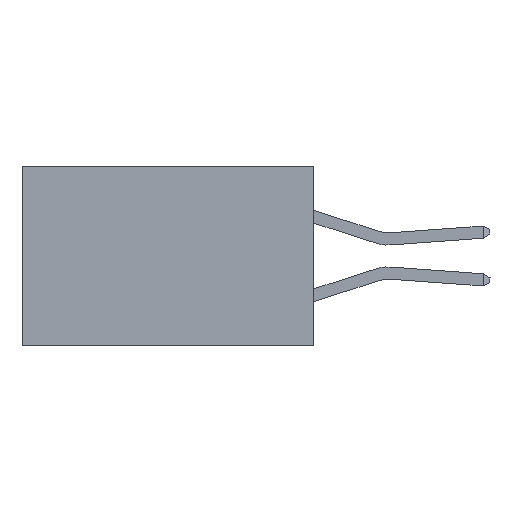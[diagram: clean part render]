
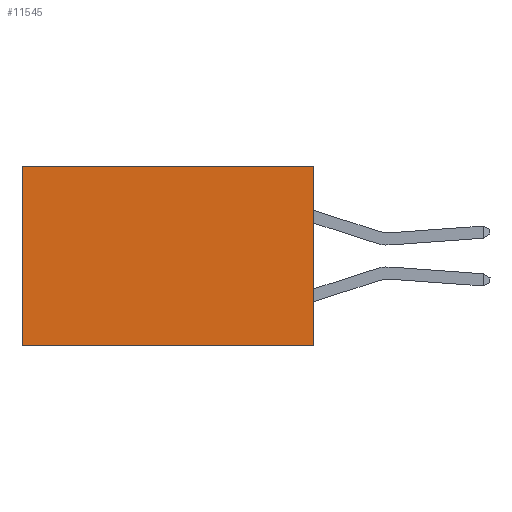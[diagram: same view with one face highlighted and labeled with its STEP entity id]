
A CAD part, left-side view. The second image highlights one B-rep face of the part: STEP entity #11545.
In plain terms, the highlighted planar face has unit normal (-1, 0, 0).
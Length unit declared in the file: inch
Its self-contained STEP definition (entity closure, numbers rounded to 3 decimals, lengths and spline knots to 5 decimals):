
#712 = ORIENTED_EDGE ( 'NONE', *, *, #10386, .T. ) ;
#1958 = CARTESIAN_POINT ( 'NONE',  ( 0.2875, 0.6, 0. ) ) ;
#3313 = ORIENTED_EDGE ( 'NONE', *, *, #13810, .F. ) ;
#3644 = LINE ( 'NONE', #19814, #23081 ) ;
#4538 = VECTOR ( 'NONE', #5929, 39.37008 ) ;
#5320 = DIRECTION ( 'NONE',  ( 1., 0., 0. ) ) ;
#5450 = ORIENTED_EDGE ( 'NONE', *, *, #22637, .T. ) ;
#5929 = DIRECTION ( 'NONE',  ( 0., 0., -1. ) ) ;
#6014 = CARTESIAN_POINT ( 'NONE',  ( 0.2875, 0., 0. ) ) ;
#7818 = EDGE_CURVE ( 'NONE', #17699, #22112, #12250, .T. ) ;
#9010 = DIRECTION ( 'NONE',  ( 0., 1., 0. ) ) ;
#10386 = EDGE_CURVE ( 'NONE', #18219, #22112, #10652, .T. ) ;
#10652 = LINE ( 'NONE', #1958, #19691 ) ;
#11545 = ADVANCED_FACE ( 'NONE', ( #23475 ), #21593, .F. ) ;
#11817 = DIRECTION ( 'NONE',  ( 0., 1., 0. ) ) ;
#12250 = LINE ( 'NONE', #22729, #16512 ) ;
#12575 = VERTEX_POINT ( 'NONE', #23031 ) ;
#12953 = CARTESIAN_POINT ( 'NONE',  ( 0.2875, 0., -0.37 ) ) ;
#13810 = EDGE_CURVE ( 'NONE', #12575, #17699, #17866, .T. ) ;
#14348 = CARTESIAN_POINT ( 'NONE',  ( 0.2875, 0., 0. ) ) ;
#15275 = ORIENTED_EDGE ( 'NONE', *, *, #7818, .F. ) ;
#16512 = VECTOR ( 'NONE', #11817, 39.37008 ) ;
#16544 = DIRECTION ( 'NONE',  ( 0., 0., -1. ) ) ;
#17699 = VERTEX_POINT ( 'NONE', #12953 ) ;
#17785 = AXIS2_PLACEMENT_3D ( 'NONE', #14348, #5320, #17991 ) ;
#17866 = LINE ( 'NONE', #6014, #4538 ) ;
#17991 = DIRECTION ( 'NONE',  ( 0., 0., -1. ) ) ;
#18219 = VERTEX_POINT ( 'NONE', #23655 ) ;
#19522 = CARTESIAN_POINT ( 'NONE',  ( 0.2875, 0.6, -0.37 ) ) ;
#19691 = VECTOR ( 'NONE', #16544, 39.37008 ) ;
#19718 = EDGE_LOOP ( 'NONE', ( #712, #15275, #3313, #5450 ) ) ;
#19814 = CARTESIAN_POINT ( 'NONE',  ( 0.2875, 0., 0. ) ) ;
#21593 = PLANE ( 'NONE',  #17785 ) ;
#22112 = VERTEX_POINT ( 'NONE', #19522 ) ;
#22637 = EDGE_CURVE ( 'NONE', #12575, #18219, #3644, .T. ) ;
#22729 = CARTESIAN_POINT ( 'NONE',  ( 0.2875, 0., -0.37 ) ) ;
#23031 = CARTESIAN_POINT ( 'NONE',  ( 0.2875, 0., 0. ) ) ;
#23081 = VECTOR ( 'NONE', #9010, 39.37008 ) ;
#23475 = FACE_OUTER_BOUND ( 'NONE', #19718, .T. ) ;
#23655 = CARTESIAN_POINT ( 'NONE',  ( 0.2875, 0.6, 0. ) ) ;
